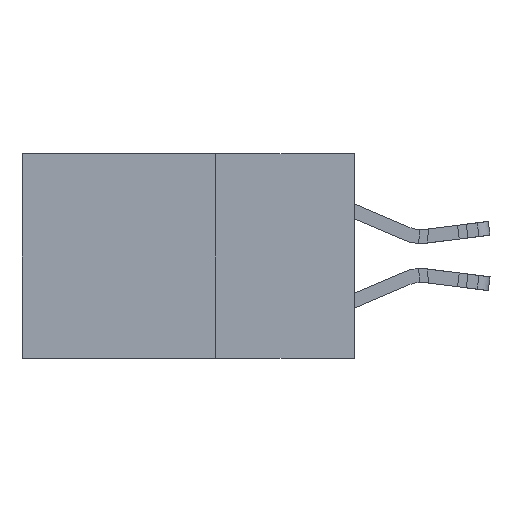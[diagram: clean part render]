
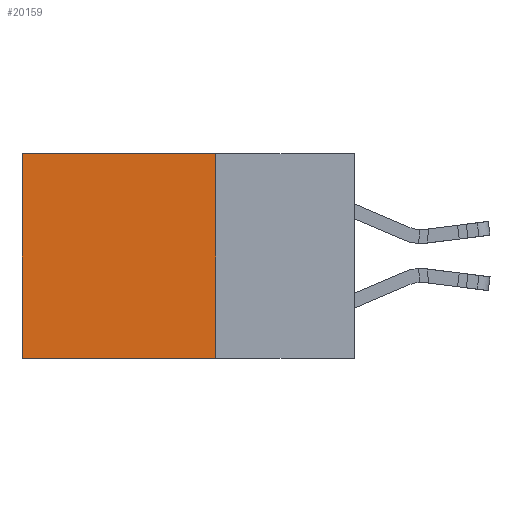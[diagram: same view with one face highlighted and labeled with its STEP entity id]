
A CAD part, left-side view. The second image highlights one B-rep face of the part: STEP entity #20159.
In plain terms, the highlighted planar face has unit normal (-1, 0, 0).
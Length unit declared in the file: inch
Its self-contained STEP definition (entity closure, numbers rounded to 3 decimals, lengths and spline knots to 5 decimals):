
#172 = CARTESIAN_POINT ( 'NONE',  ( 0.2615, 0.25, -0.37 ) ) ;
#1070 = VERTEX_POINT ( 'NONE', #14059 ) ;
#2158 = EDGE_CURVE ( 'NONE', #5656, #1070, #23806, .T. ) ;
#2261 = PLANE ( 'NONE',  #22171 ) ;
#2941 = ORIENTED_EDGE ( 'NONE', *, *, #2158, .T. ) ;
#3668 = DIRECTION ( 'NONE',  ( 0., 0., -1. ) ) ;
#3774 = CARTESIAN_POINT ( 'NONE',  ( 0.2615, 0.6, 0. ) ) ;
#4126 = DIRECTION ( 'NONE',  ( 0., 0., -1. ) ) ;
#4223 = CARTESIAN_POINT ( 'NONE',  ( 0.2615, 0.25, -0.37 ) ) ;
#4358 = ORIENTED_EDGE ( 'NONE', *, *, #12460, .F. ) ;
#4374 = VECTOR ( 'NONE', #4126, 39.37008 ) ;
#5586 = LINE ( 'NONE', #13806, #14924 ) ;
#5656 = VERTEX_POINT ( 'NONE', #3774 ) ;
#6143 = DIRECTION ( 'NONE',  ( 1., 0., 0. ) ) ;
#6957 = VERTEX_POINT ( 'NONE', #12740 ) ;
#8262 = CARTESIAN_POINT ( 'NONE',  ( 0.2615, 0.25, 0. ) ) ;
#8790 = ORIENTED_EDGE ( 'NONE', *, *, #22186, .F. ) ;
#8873 = EDGE_LOOP ( 'NONE', ( #2941, #4358, #8790, #15595 ) ) ;
#12055 = DIRECTION ( 'NONE',  ( 0., 1., 0. ) ) ;
#12460 = EDGE_CURVE ( 'NONE', #6957, #1070, #5586, .T. ) ;
#12740 = CARTESIAN_POINT ( 'NONE',  ( 0.2615, 0.25, -0.37 ) ) ;
#13806 = CARTESIAN_POINT ( 'NONE',  ( 0.2615, 0.25, -0.37 ) ) ;
#13938 = CARTESIAN_POINT ( 'NONE',  ( 0.2615, 0.25, 0. ) ) ;
#14059 = CARTESIAN_POINT ( 'NONE',  ( 0.2615, 0.6, -0.37 ) ) ;
#14730 = FACE_OUTER_BOUND ( 'NONE', #8873, .T. ) ;
#14924 = VECTOR ( 'NONE', #15675, 39.37008 ) ;
#15510 = CARTESIAN_POINT ( 'NONE',  ( 0.2615, 0.6, -0.37 ) ) ;
#15595 = ORIENTED_EDGE ( 'NONE', *, *, #19655, .T. ) ;
#15675 = DIRECTION ( 'NONE',  ( 0., 1., 0. ) ) ;
#19102 = DIRECTION ( 'NONE',  ( 0., 0., -1. ) ) ;
#19631 = VECTOR ( 'NONE', #12055, 39.37008 ) ;
#19655 = EDGE_CURVE ( 'NONE', #20885, #5656, #20209, .T. ) ;
#20159 = ADVANCED_FACE ( 'NONE', ( #14730 ), #2261, .F. ) ;
#20209 = LINE ( 'NONE', #13938, #19631 ) ;
#20885 = VERTEX_POINT ( 'NONE', #8262 ) ;
#22171 = AXIS2_PLACEMENT_3D ( 'NONE', #4223, #6143, #19102 ) ;
#22186 = EDGE_CURVE ( 'NONE', #20885, #6957, #23553, .T. ) ;
#23241 = VECTOR ( 'NONE', #3668, 39.37008 ) ;
#23553 = LINE ( 'NONE', #172, #4374 ) ;
#23806 = LINE ( 'NONE', #15510, #23241 ) ;
